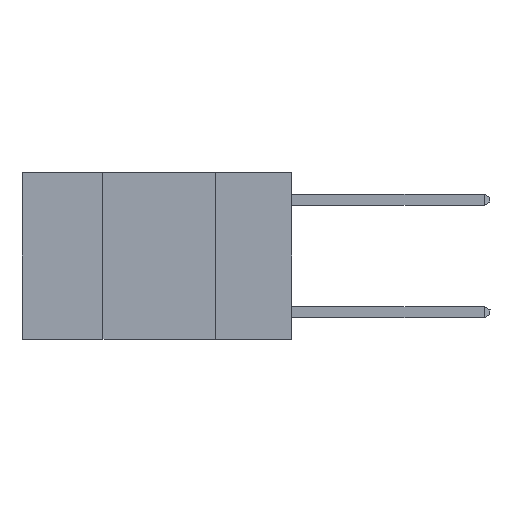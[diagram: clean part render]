
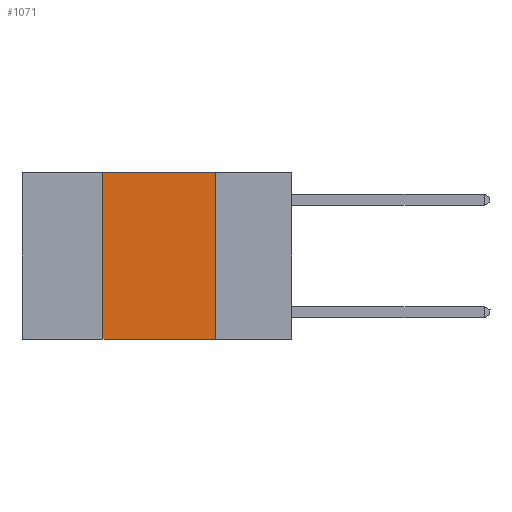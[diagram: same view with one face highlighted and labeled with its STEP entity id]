
A CAD part, left-side view. The second image highlights one B-rep face of the part: STEP entity #1071.
In plain terms, the highlighted planar face has unit normal (-1, 0, 0).
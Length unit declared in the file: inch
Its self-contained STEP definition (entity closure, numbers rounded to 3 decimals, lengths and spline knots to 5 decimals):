
#81 = ORIENTED_EDGE ( 'NONE', *, *, #2351, .F. ) ;
#813 = EDGE_CURVE ( 'NONE', #9577, #9914, #1774, .T. ) ;
#1071 = ADVANCED_FACE ( 'NONE', ( #2723 ), #10259, .F. ) ;
#1774 = LINE ( 'NONE', #2026, #5896 ) ;
#1912 = EDGE_CURVE ( 'NONE', #4524, #9914, #10363, .T. ) ;
#2026 = CARTESIAN_POINT ( 'NONE',  ( 0., 0.17, 0. ) ) ;
#2295 = VECTOR ( 'NONE', #11263, 39.37008 ) ;
#2351 = EDGE_CURVE ( 'NONE', #9627, #9577, #5317, .T. ) ;
#2611 = VECTOR ( 'NONE', #4348, 39.37008 ) ;
#2723 = FACE_OUTER_BOUND ( 'NONE', #7963, .T. ) ;
#2855 = CARTESIAN_POINT ( 'NONE',  ( 0., 0.42, 0. ) ) ;
#4065 = CARTESIAN_POINT ( 'NONE',  ( 0., 0.6, -0.37 ) ) ;
#4348 = DIRECTION ( 'NONE',  ( 0., -1., 0. ) ) ;
#4418 = VECTOR ( 'NONE', #9899, 39.37008 ) ;
#4427 = ORIENTED_EDGE ( 'NONE', *, *, #1912, .T. ) ;
#4470 = CARTESIAN_POINT ( 'NONE',  ( 0., 0.6, 0. ) ) ;
#4497 = CARTESIAN_POINT ( 'NONE',  ( 0., 0.6, 0. ) ) ;
#4524 = VERTEX_POINT ( 'NONE', #11511 ) ;
#5317 = LINE ( 'NONE', #4470, #2611 ) ;
#5475 = CARTESIAN_POINT ( 'NONE',  ( 0., 0.42, 0. ) ) ;
#5896 = VECTOR ( 'NONE', #8888, 39.37008 ) ;
#6453 = CARTESIAN_POINT ( 'NONE',  ( 0., 0.17, 0. ) ) ;
#6469 = LINE ( 'NONE', #2855, #4418 ) ;
#6482 = AXIS2_PLACEMENT_3D ( 'NONE', #4497, #9728, #8630 ) ;
#6983 = CARTESIAN_POINT ( 'NONE',  ( 0., 0.17, -0.37 ) ) ;
#7963 = EDGE_LOOP ( 'NONE', ( #8826, #81, #8540, #4427 ) ) ;
#8540 = ORIENTED_EDGE ( 'NONE', *, *, #9850, .F. ) ;
#8630 = DIRECTION ( 'NONE',  ( 0., 0., -1. ) ) ;
#8826 = ORIENTED_EDGE ( 'NONE', *, *, #813, .F. ) ;
#8888 = DIRECTION ( 'NONE',  ( 0., 0., -1. ) ) ;
#9577 = VERTEX_POINT ( 'NONE', #6453 ) ;
#9627 = VERTEX_POINT ( 'NONE', #5475 ) ;
#9728 = DIRECTION ( 'NONE',  ( 1., 0., 0. ) ) ;
#9850 = EDGE_CURVE ( 'NONE', #4524, #9627, #6469, .T. ) ;
#9899 = DIRECTION ( 'NONE',  ( 0., 0., 1. ) ) ;
#9914 = VERTEX_POINT ( 'NONE', #6983 ) ;
#10259 = PLANE ( 'NONE',  #6482 ) ;
#10363 = LINE ( 'NONE', #4065, #2295 ) ;
#11263 = DIRECTION ( 'NONE',  ( 0., -1., 0. ) ) ;
#11511 = CARTESIAN_POINT ( 'NONE',  ( 0., 0.42, -0.37 ) ) ;
